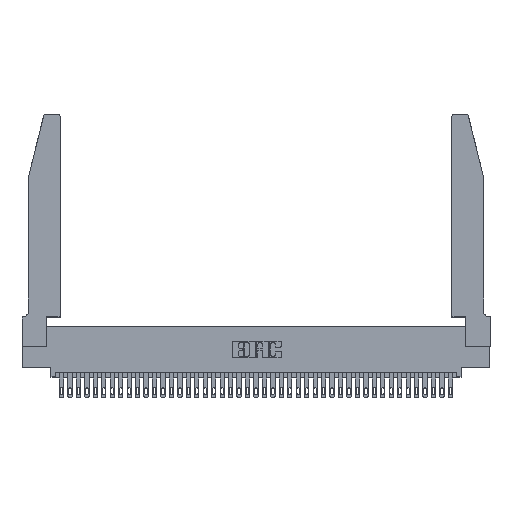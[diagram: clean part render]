
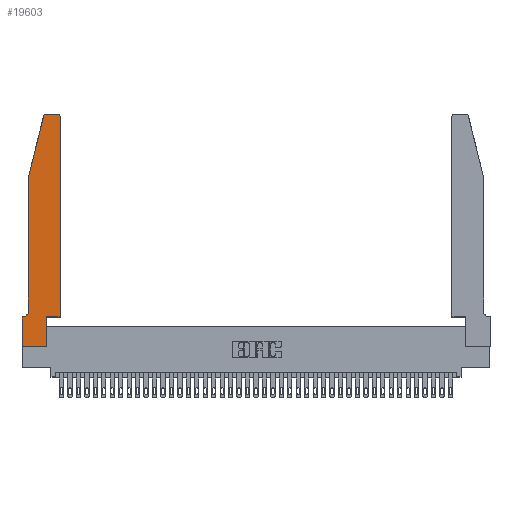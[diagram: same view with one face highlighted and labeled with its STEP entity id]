
A CAD part, top view. The second image highlights one B-rep face of the part: STEP entity #19603.
In plain terms, the highlighted planar face has unit normal (0, 0, 1).
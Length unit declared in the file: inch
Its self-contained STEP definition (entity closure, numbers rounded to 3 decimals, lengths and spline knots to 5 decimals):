
#20 = CARTESIAN_POINT ( 'NONE',  ( 0.4505, 0.35, 0.37 ) ) ;
#271 = EDGE_LOOP ( 'NONE', ( #4859, #2086, #3550, #18936, #13924, #1784, #19630, #32774, #35789, #39594, #3896, #8254 ) ) ;
#336 = DIRECTION ( 'NONE',  ( 1., 0., 0. ) ) ;
#466 = LINE ( 'NONE', #1624, #32175 ) ;
#483 = CARTESIAN_POINT ( 'NONE',  ( 0.4205, 2.72, 0.37 ) ) ;
#1151 = DIRECTION ( 'NONE',  ( -1., 0., 0. ) ) ;
#1624 = CARTESIAN_POINT ( 'NONE',  ( 0.4505, 0.35, 0.37 ) ) ;
#1784 = ORIENTED_EDGE ( 'NONE', *, *, #29322, .T. ) ;
#1959 = AXIS2_PLACEMENT_3D ( 'NONE', #24559, #37183, #30653 ) ;
#2086 = ORIENTED_EDGE ( 'NONE', *, *, #32097, .T. ) ;
#3410 = LINE ( 'NONE', #17877, #37057 ) ;
#3550 = ORIENTED_EDGE ( 'NONE', *, *, #3746, .T. ) ;
#3746 = EDGE_CURVE ( 'NONE', #13458, #28908, #15952, .T. ) ;
#3896 = ORIENTED_EDGE ( 'NONE', *, *, #5258, .T. ) ;
#4229 = EDGE_CURVE ( 'NONE', #16642, #36903, #5564, .T. ) ;
#4859 = ORIENTED_EDGE ( 'NONE', *, *, #5454, .T. ) ;
#5258 = EDGE_CURVE ( 'NONE', #31583, #18944, #466, .T. ) ;
#5454 = EDGE_CURVE ( 'NONE', #22799, #23479, #37709, .T. ) ;
#5564 = LINE ( 'NONE', #13326, #10993 ) ;
#6017 = VERTEX_POINT ( 'NONE', #24286 ) ;
#6524 = AXIS2_PLACEMENT_3D ( 'NONE', #10238, #25826, #336 ) ;
#6827 = CARTESIAN_POINT ( 'NONE',  ( 0.2865, 0.35, 0.37 ) ) ;
#7489 = CIRCLE ( 'NONE', #10322, 0.03 ) ;
#8254 = ORIENTED_EDGE ( 'NONE', *, *, #38305, .T. ) ;
#9845 = CARTESIAN_POINT ( 'NONE',  ( 0.2865, 0., 0.37 ) ) ;
#10238 = CARTESIAN_POINT ( 'NONE',  ( 0.284, 2.72, 0.37 ) ) ;
#10322 = AXIS2_PLACEMENT_3D ( 'NONE', #483, #32377, #35565 ) ;
#10589 = DIRECTION ( 'NONE',  ( 0., -1., 0. ) ) ;
#10739 = CARTESIAN_POINT ( 'NONE',  ( 0., 0., 0.37 ) ) ;
#10993 = VECTOR ( 'NONE', #10589, 39.37008 ) ;
#11601 = CARTESIAN_POINT ( 'NONE',  ( 0.2865, 0.35, 0.37 ) ) ;
#12160 = DIRECTION ( 'NONE',  ( 0., 0., 1. ) ) ;
#13326 = CARTESIAN_POINT ( 'NONE',  ( 0., 0., 0.37 ) ) ;
#13458 = VERTEX_POINT ( 'NONE', #17994 ) ;
#13549 = VERTEX_POINT ( 'NONE', #11601 ) ;
#13924 = ORIENTED_EDGE ( 'NONE', *, *, #17542, .T. ) ;
#14400 = EDGE_CURVE ( 'NONE', #29654, #13549, #36502, .T. ) ;
#14460 = VECTOR ( 'NONE', #19376, 39.37008 ) ;
#14841 = CARTESIAN_POINT ( 'NONE',  ( 0.4505, 0.35, 0.37 ) ) ;
#14851 = CARTESIAN_POINT ( 'NONE',  ( 0.0755, 0.42, 0.37 ) ) ;
#15952 = LINE ( 'NONE', #34853, #14460 ) ;
#16642 = VERTEX_POINT ( 'NONE', #17852 ) ;
#16721 = FACE_OUTER_BOUND ( 'NONE', #271, .T. ) ;
#17170 = DIRECTION ( 'NONE',  ( 1., 0., 0. ) ) ;
#17542 = EDGE_CURVE ( 'NONE', #17566, #6017, #23823, .T. ) ;
#17566 = VERTEX_POINT ( 'NONE', #14851 ) ;
#17852 = CARTESIAN_POINT ( 'NONE',  ( 0., 0.35, 0.37 ) ) ;
#17877 = CARTESIAN_POINT ( 'NONE',  ( 0.0755, 2., 0.37 ) ) ;
#17994 = CARTESIAN_POINT ( 'NONE',  ( 0.25487, 2.72718, 0.37 ) ) ;
#18153 = DIRECTION ( 'NONE',  ( 1., 0., 0. ) ) ;
#18164 = DIRECTION ( 'NONE',  ( 1., 0., 0. ) ) ;
#18446 = DIRECTION ( 'NONE',  ( 0., -1., 0. ) ) ;
#18936 = ORIENTED_EDGE ( 'NONE', *, *, #19647, .T. ) ;
#18944 = VERTEX_POINT ( 'NONE', #28186 ) ;
#19376 = DIRECTION ( 'NONE',  ( -0.239, -0.971, 0. ) ) ;
#19603 = ADVANCED_FACE ( 'NONE', ( #16721 ), #20354, .T. ) ;
#19630 = ORIENTED_EDGE ( 'NONE', *, *, #4229, .T. ) ;
#19647 = EDGE_CURVE ( 'NONE', #28908, #17566, #3410, .T. ) ;
#19804 = VECTOR ( 'NONE', #17170, 39.37008 ) ;
#20354 = PLANE ( 'NONE',  #20496 ) ;
#20496 = AXIS2_PLACEMENT_3D ( 'NONE', #33165, #12160, #18164 ) ;
#20575 = LINE ( 'NONE', #14841, #26578 ) ;
#21085 = DIRECTION ( 'NONE',  ( 0., 1., 0. ) ) ;
#21772 = EDGE_CURVE ( 'NONE', #13549, #31583, #20575, .T. ) ;
#22799 = VERTEX_POINT ( 'NONE', #38400 ) ;
#22819 = DIRECTION ( 'NONE',  ( 0., 1., 0. ) ) ;
#23479 = VERTEX_POINT ( 'NONE', #26625 ) ;
#23823 = CIRCLE ( 'NONE', #1959, 0.07 ) ;
#24286 = CARTESIAN_POINT ( 'NONE',  ( 0.0055, 0.35, 0.37 ) ) ;
#24559 = CARTESIAN_POINT ( 'NONE',  ( 0.0055, 0.42, 0.37 ) ) ;
#25109 = CARTESIAN_POINT ( 'NONE',  ( 0.0755, 2., 0.37 ) ) ;
#25826 = DIRECTION ( 'NONE',  ( 0., 0., 1. ) ) ;
#26578 = VECTOR ( 'NONE', #18153, 39.37008 ) ;
#26625 = CARTESIAN_POINT ( 'NONE',  ( 0.284, 2.75, 0.37 ) ) ;
#28186 = CARTESIAN_POINT ( 'NONE',  ( 0.4505, 2.72, 0.37 ) ) ;
#28381 = CIRCLE ( 'NONE', #6524, 0.03 ) ;
#28908 = VERTEX_POINT ( 'NONE', #25109 ) ;
#29322 = EDGE_CURVE ( 'NONE', #6017, #16642, #32029, .T. ) ;
#29654 = VERTEX_POINT ( 'NONE', #9845 ) ;
#30518 = VECTOR ( 'NONE', #22819, 39.37008 ) ;
#30653 = DIRECTION ( 'NONE',  ( -1., 0., 0. ) ) ;
#30881 = CARTESIAN_POINT ( 'NONE',  ( 0.0755, 0.35, 0.37 ) ) ;
#31575 = VECTOR ( 'NONE', #40170, 39.37008 ) ;
#31583 = VERTEX_POINT ( 'NONE', #20 ) ;
#32029 = LINE ( 'NONE', #30881, #31575 ) ;
#32097 = EDGE_CURVE ( 'NONE', #23479, #13458, #28381, .T. ) ;
#32175 = VECTOR ( 'NONE', #21085, 39.37008 ) ;
#32377 = DIRECTION ( 'NONE',  ( 0., 0., 1. ) ) ;
#32774 = ORIENTED_EDGE ( 'NONE', *, *, #32939, .T. ) ;
#32939 = EDGE_CURVE ( 'NONE', #36903, #29654, #36729, .T. ) ;
#33165 = CARTESIAN_POINT ( 'NONE',  ( 0., 0.35, 0.37 ) ) ;
#34853 = CARTESIAN_POINT ( 'NONE',  ( 0.0755, 2., 0.37 ) ) ;
#35565 = DIRECTION ( 'NONE',  ( 1., 0., 0. ) ) ;
#35789 = ORIENTED_EDGE ( 'NONE', *, *, #14400, .T. ) ;
#36422 = CARTESIAN_POINT ( 'NONE',  ( 0., 0., 0.37 ) ) ;
#36502 = LINE ( 'NONE', #6827, #30518 ) ;
#36729 = LINE ( 'NONE', #10739, #19804 ) ;
#36903 = VERTEX_POINT ( 'NONE', #36422 ) ;
#37057 = VECTOR ( 'NONE', #18446, 39.37008 ) ;
#37183 = DIRECTION ( 'NONE',  ( 0., 0., -1. ) ) ;
#37709 = LINE ( 'NONE', #40709, #40692 ) ;
#38305 = EDGE_CURVE ( 'NONE', #18944, #22799, #7489, .T. ) ;
#38400 = CARTESIAN_POINT ( 'NONE',  ( 0.4205, 2.75, 0.37 ) ) ;
#39594 = ORIENTED_EDGE ( 'NONE', *, *, #21772, .T. ) ;
#40170 = DIRECTION ( 'NONE',  ( -1., 0., 0. ) ) ;
#40692 = VECTOR ( 'NONE', #1151, 39.37008 ) ;
#40709 = CARTESIAN_POINT ( 'NONE',  ( 0.2605, 2.75, 0.37 ) ) ;
